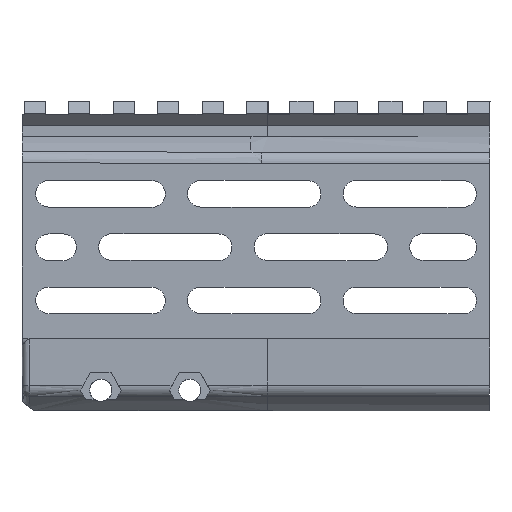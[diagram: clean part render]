
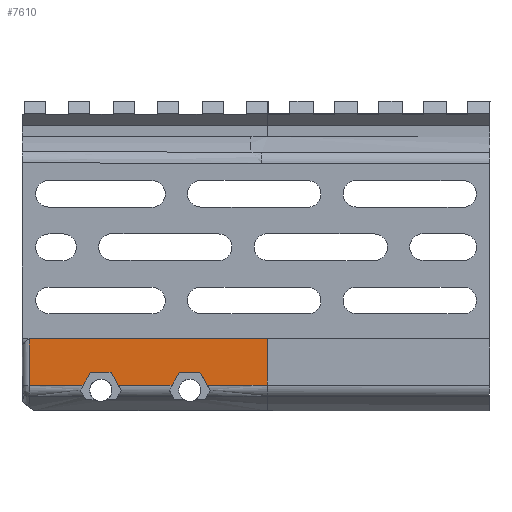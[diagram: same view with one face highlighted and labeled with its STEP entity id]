
A CAD part, front view. The second image highlights one B-rep face of the part: STEP entity #7610.
In plain terms, the highlighted planar face has unit normal (0, -1, 0).
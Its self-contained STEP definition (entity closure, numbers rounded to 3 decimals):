
#282=PLANE('',#8040);
#579=FACE_OUTER_BOUND('',#977,.T.);
#977=EDGE_LOOP('',(#5452,#5453,#5454,#5455,#5456,#5457,#5458,#5459,#5460,
#5461,#5462,#5463,#5464,#5465));
#1475=LINE('',#11176,#2361);
#1480=LINE('',#11212,#2366);
#1486=LINE('',#11230,#2372);
#1489=LINE('',#11264,#2375);
#1494=LINE('',#11300,#2380);
#1500=LINE('',#11325,#2386);
#1502=LINE('',#11355,#2388);
#1503=LINE('',#11357,#2389);
#1504=LINE('',#11359,#2390);
#1505=LINE('',#11361,#2391);
#1506=LINE('',#11363,#2392);
#1507=LINE('',#11365,#2393);
#1508=LINE('',#11367,#2394);
#1509=LINE('',#11368,#2395);
#2361=VECTOR('',#8678,10.);
#2366=VECTOR('',#8687,10.);
#2372=VECTOR('',#8695,10.);
#2375=VECTOR('',#8708,10.);
#2380=VECTOR('',#8717,10.);
#2386=VECTOR('',#8725,10.);
#2388=VECTOR('',#8737,10.);
#2389=VECTOR('',#8738,10.);
#2390=VECTOR('',#8739,10.);
#2391=VECTOR('',#8740,10.);
#2392=VECTOR('',#8741,10.);
#2393=VECTOR('',#8742,10.);
#2394=VECTOR('',#8743,10.);
#2395=VECTOR('',#8744,10.);
#3406=VERTEX_POINT('',#11172);
#3408=VERTEX_POINT('',#11175);
#3414=VERTEX_POINT('',#11211);
#3417=VERTEX_POINT('',#11218);
#3425=VERTEX_POINT('',#11260);
#3427=VERTEX_POINT('',#11263);
#3433=VERTEX_POINT('',#11299);
#3436=VERTEX_POINT('',#11306);
#3444=VERTEX_POINT('',#11356);
#3445=VERTEX_POINT('',#11358);
#3446=VERTEX_POINT('',#11360);
#3447=VERTEX_POINT('',#11362);
#3448=VERTEX_POINT('',#11364);
#3449=VERTEX_POINT('',#11366);
#4187=EDGE_CURVE('',#3408,#3406,#1475,.T.);
#4195=EDGE_CURVE('',#3414,#3408,#1480,.T.);
#4202=EDGE_CURVE('',#3417,#3414,#1486,.T.);
#4211=EDGE_CURVE('',#3427,#3425,#1489,.T.);
#4219=EDGE_CURVE('',#3433,#3427,#1494,.T.);
#4226=EDGE_CURVE('',#3436,#3433,#1500,.T.);
#4234=EDGE_CURVE('',#3406,#3436,#1502,.T.);
#4235=EDGE_CURVE('',#3425,#3444,#1503,.T.);
#4236=EDGE_CURVE('',#3445,#3444,#1504,.T.);
#4237=EDGE_CURVE('',#3445,#3446,#1505,.T.);
#4238=EDGE_CURVE('',#3446,#3447,#1506,.T.);
#4239=EDGE_CURVE('',#3448,#3447,#1507,.T.);
#4240=EDGE_CURVE('',#3448,#3449,#1508,.T.);
#4241=EDGE_CURVE('',#3449,#3417,#1509,.T.);
#5452=ORIENTED_EDGE('',*,*,#4202,.T.);
#5453=ORIENTED_EDGE('',*,*,#4195,.T.);
#5454=ORIENTED_EDGE('',*,*,#4187,.T.);
#5455=ORIENTED_EDGE('',*,*,#4234,.T.);
#5456=ORIENTED_EDGE('',*,*,#4226,.T.);
#5457=ORIENTED_EDGE('',*,*,#4219,.T.);
#5458=ORIENTED_EDGE('',*,*,#4211,.T.);
#5459=ORIENTED_EDGE('',*,*,#4235,.T.);
#5460=ORIENTED_EDGE('',*,*,#4236,.F.);
#5461=ORIENTED_EDGE('',*,*,#4237,.T.);
#5462=ORIENTED_EDGE('',*,*,#4238,.T.);
#5463=ORIENTED_EDGE('',*,*,#4239,.F.);
#5464=ORIENTED_EDGE('',*,*,#4240,.T.);
#5465=ORIENTED_EDGE('',*,*,#4241,.T.);
#7610=ADVANCED_FACE('',(#579),#282,.F.);
#8040=AXIS2_PLACEMENT_3D('',#11354,#8735,#8736);
#8678=DIRECTION('',(0.5,0.,-0.866));
#8687=DIRECTION('',(1.,0.,0.));
#8695=DIRECTION('',(0.5,0.,0.866));
#8708=DIRECTION('',(0.5,0.,-0.866));
#8717=DIRECTION('',(1.,0.,0.));
#8725=DIRECTION('',(0.5,0.,0.866));
#8735=DIRECTION('center_axis',(0.,1.,0.));
#8736=DIRECTION('ref_axis',(1.,0.,0.));
#8737=DIRECTION('',(1.,0.,0.002));
#8738=DIRECTION('',(1.,0.,0.002));
#8739=DIRECTION('',(-0.002,0.,-1.));
#8740=DIRECTION('',(0.002,0.,1.));
#8741=DIRECTION('',(-1.,0.,0.002));
#8742=DIRECTION('',(0.002,0.,1.));
#8743=DIRECTION('',(0.002,0.,-1.));
#8744=DIRECTION('',(1.,0.,0.002));
#11172=CARTESIAN_POINT('',(2958.726,309.834,69.312));
#11175=CARTESIAN_POINT('',(2957.049,309.834,72.217));
#11176=CARTESIAN_POINT('',(2972.134,309.834,46.089));
#11211=CARTESIAN_POINT('',(2952.43,309.834,72.217));
#11212=CARTESIAN_POINT('',(3020.592,309.834,72.217));
#11218=CARTESIAN_POINT('',(2950.745,309.834,69.298));
#11230=CARTESIAN_POINT('',(2969.694,309.834,102.119));
#11260=CARTESIAN_POINT('',(2978.706,309.834,69.347));
#11263=CARTESIAN_POINT('',(2977.049,309.834,72.217));
#11264=CARTESIAN_POINT('',(2989.634,309.834,50.419));
#11299=CARTESIAN_POINT('',(2972.43,309.834,72.217));
#11300=CARTESIAN_POINT('',(3030.592,309.834,72.217));
#11306=CARTESIAN_POINT('',(2970.765,309.834,69.333));
#11325=CARTESIAN_POINT('',(2987.194,309.834,97.789));
#11354=CARTESIAN_POINT('Origin',(3088.754,309.834,78.582));
#11355=CARTESIAN_POINT('',(2986.642,309.834,69.361));
#11356=CARTESIAN_POINT('',(2992.179,309.834,69.37));
#11357=CARTESIAN_POINT('',(2986.642,309.834,69.361));
#11358=CARTESIAN_POINT('',(2992.197,309.834,79.65));
#11359=CARTESIAN_POINT('',(2992.212,309.834,88.495));
#11360=CARTESIAN_POINT('',(2992.197,309.834,79.838));
#11361=CARTESIAN_POINT('',(2992.197,309.834,79.65));
#11362=CARTESIAN_POINT('',(2938.611,309.834,79.931));
#11363=CARTESIAN_POINT('',(2939.823,309.834,79.929));
#11364=CARTESIAN_POINT('',(2938.611,309.834,79.743));
#11365=CARTESIAN_POINT('',(2938.611,309.834,79.743));
#11366=CARTESIAN_POINT('',(2938.629,309.834,69.277));
#11367=CARTESIAN_POINT('',(2938.616,309.834,76.91));
#11368=CARTESIAN_POINT('',(2986.642,309.834,69.361));
